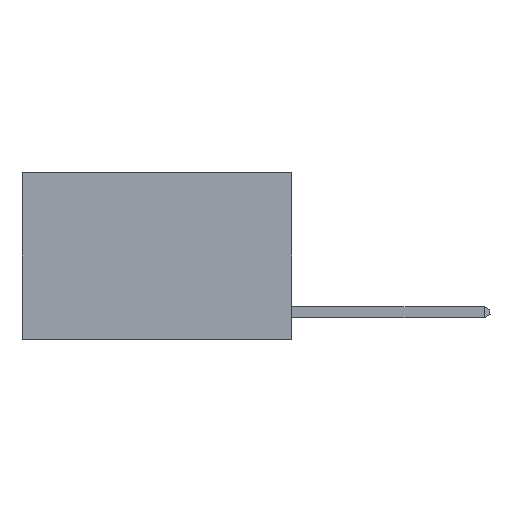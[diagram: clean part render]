
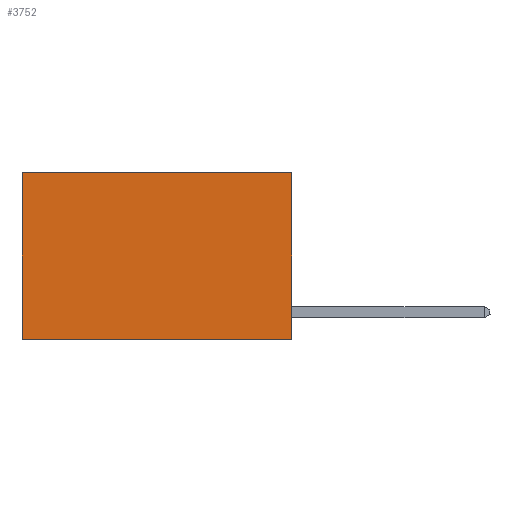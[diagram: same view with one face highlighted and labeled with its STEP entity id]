
A CAD part, left-side view. The second image highlights one B-rep face of the part: STEP entity #3752.
In plain terms, the highlighted planar face has unit normal (-1, 0, 0).
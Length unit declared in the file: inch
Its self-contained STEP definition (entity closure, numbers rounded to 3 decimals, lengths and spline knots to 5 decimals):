
#186 = LINE ( 'NONE', #10092, #5523 ) ;
#773 = CARTESIAN_POINT ( 'NONE',  ( 0.2625, 0., 0. ) ) ;
#1419 = CARTESIAN_POINT ( 'NONE',  ( 0.2625, 0.6, 0. ) ) ;
#1746 = EDGE_CURVE ( 'NONE', #7334, #18581, #9681, .T. ) ;
#2456 = DIRECTION ( 'NONE',  ( 0., 0., -1. ) ) ;
#2544 = EDGE_CURVE ( 'NONE', #7334, #21337, #186, .T. ) ;
#2683 = EDGE_CURVE ( 'NONE', #18581, #8145, #14809, .T. ) ;
#3178 = CARTESIAN_POINT ( 'NONE',  ( 0.2625, 0.6, -0.37 ) ) ;
#3539 = AXIS2_PLACEMENT_3D ( 'NONE', #773, #20136, #2456 ) ;
#3752 = ADVANCED_FACE ( 'NONE', ( #20019 ), #8368, .F. ) ;
#3908 = ORIENTED_EDGE ( 'NONE', *, *, #2683, .F. ) ;
#4824 = ORIENTED_EDGE ( 'NONE', *, *, #15316, .T. ) ;
#5523 = VECTOR ( 'NONE', #23648, 39.37008 ) ;
#7334 = VERTEX_POINT ( 'NONE', #23146 ) ;
#7822 = LINE ( 'NONE', #8068, #14604 ) ;
#8068 = CARTESIAN_POINT ( 'NONE',  ( 0.2625, 0.6, 0. ) ) ;
#8145 = VERTEX_POINT ( 'NONE', #3178 ) ;
#8197 = DIRECTION ( 'NONE',  ( 0., 0., -1. ) ) ;
#8368 = PLANE ( 'NONE',  #3539 ) ;
#9681 = LINE ( 'NONE', #15544, #10024 ) ;
#10024 = VECTOR ( 'NONE', #13501, 39.37008 ) ;
#10092 = CARTESIAN_POINT ( 'NONE',  ( 0.2625, 0., 0. ) ) ;
#11002 = CARTESIAN_POINT ( 'NONE',  ( 0.2625, 0., -0.37 ) ) ;
#12964 = EDGE_LOOP ( 'NONE', ( #4824, #3908, #19611, #24162 ) ) ;
#13501 = DIRECTION ( 'NONE',  ( 0., 0., -1. ) ) ;
#14604 = VECTOR ( 'NONE', #8197, 39.37008 ) ;
#14809 = LINE ( 'NONE', #11002, #19484 ) ;
#15316 = EDGE_CURVE ( 'NONE', #21337, #8145, #7822, .T. ) ;
#15544 = CARTESIAN_POINT ( 'NONE',  ( 0.2625, 0., 0. ) ) ;
#18581 = VERTEX_POINT ( 'NONE', #23937 ) ;
#19484 = VECTOR ( 'NONE', #24301, 39.37008 ) ;
#19611 = ORIENTED_EDGE ( 'NONE', *, *, #1746, .F. ) ;
#20019 = FACE_OUTER_BOUND ( 'NONE', #12964, .T. ) ;
#20136 = DIRECTION ( 'NONE',  ( 1., 0., 0. ) ) ;
#21337 = VERTEX_POINT ( 'NONE', #1419 ) ;
#23146 = CARTESIAN_POINT ( 'NONE',  ( 0.2625, 0., 0. ) ) ;
#23648 = DIRECTION ( 'NONE',  ( 0., 1., 0. ) ) ;
#23937 = CARTESIAN_POINT ( 'NONE',  ( 0.2625, 0., -0.37 ) ) ;
#24162 = ORIENTED_EDGE ( 'NONE', *, *, #2544, .T. ) ;
#24301 = DIRECTION ( 'NONE',  ( 0., 1., 0. ) ) ;
